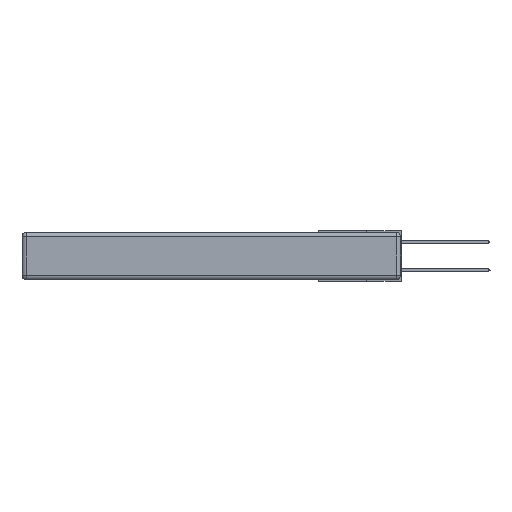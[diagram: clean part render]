
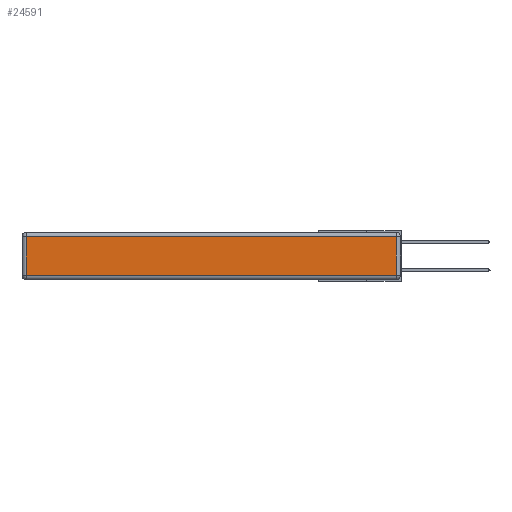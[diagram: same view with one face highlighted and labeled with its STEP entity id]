
A CAD part, left-side view. The second image highlights one B-rep face of the part: STEP entity #24591.
In plain terms, the highlighted planar face has unit normal (-1, 0, 0).
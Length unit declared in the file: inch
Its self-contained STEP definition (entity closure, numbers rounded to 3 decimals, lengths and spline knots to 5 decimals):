
#1178 = LINE ( 'NONE', #32410, #7089 ) ;
#2088 = CARTESIAN_POINT ( 'NONE',  ( 0., 0.03, -0.343 ) ) ;
#2269 = DIRECTION ( 'NONE',  ( 0., 0., -1. ) ) ;
#2375 = ORIENTED_EDGE ( 'NONE', *, *, #16801, .T. ) ;
#3249 = VERTEX_POINT ( 'NONE', #9468 ) ;
#5847 = DIRECTION ( 'NONE',  ( 0., 0., 1. ) ) ;
#6682 = DIRECTION ( 'NONE',  ( 0., -1., 0. ) ) ;
#7089 = VECTOR ( 'NONE', #22239, 39.37008 ) ;
#7823 = DIRECTION ( 'NONE',  ( -1., 0., 0. ) ) ;
#9468 = CARTESIAN_POINT ( 'NONE',  ( 0., 0.03, -0.313 ) ) ;
#9846 = EDGE_CURVE ( 'NONE', #3249, #24223, #26420, .T. ) ;
#10158 = VECTOR ( 'NONE', #27763, 39.37008 ) ;
#10250 = PLANE ( 'NONE',  #26780 ) ;
#10438 = EDGE_LOOP ( 'NONE', ( #25414, #20295, #2375, #22472 ) ) ;
#11338 = LINE ( 'NONE', #29591, #30744 ) ;
#11528 = LINE ( 'NONE', #15069, #28571 ) ;
#12261 = EDGE_CURVE ( 'NONE', #16256, #3249, #11338, .T. ) ;
#13826 = CARTESIAN_POINT ( 'NONE',  ( 0., 2.72, -0.03 ) ) ;
#15061 = CARTESIAN_POINT ( 'NONE',  ( 0., 2.72, -0.313 ) ) ;
#15069 = CARTESIAN_POINT ( 'NONE',  ( 0., 2.72, -0.343 ) ) ;
#16256 = VERTEX_POINT ( 'NONE', #15061 ) ;
#16801 = EDGE_CURVE ( 'NONE', #24223, #30823, #1178, .T. ) ;
#20295 = ORIENTED_EDGE ( 'NONE', *, *, #9846, .T. ) ;
#22239 = DIRECTION ( 'NONE',  ( 0., 1., 0. ) ) ;
#22472 = ORIENTED_EDGE ( 'NONE', *, *, #23863, .T. ) ;
#23811 = CARTESIAN_POINT ( 'NONE',  ( 0., 0.03, -0.03 ) ) ;
#23863 = EDGE_CURVE ( 'NONE', #30823, #16256, #11528, .T. ) ;
#24223 = VERTEX_POINT ( 'NONE', #23811 ) ;
#24591 = ADVANCED_FACE ( 'NONE', ( #32440 ), #10250, .T. ) ;
#25414 = ORIENTED_EDGE ( 'NONE', *, *, #12261, .T. ) ;
#26420 = LINE ( 'NONE', #2088, #10158 ) ;
#26780 = AXIS2_PLACEMENT_3D ( 'NONE', #27995, #7823, #5847 ) ;
#27763 = DIRECTION ( 'NONE',  ( 0., 0., 1. ) ) ;
#27995 = CARTESIAN_POINT ( 'NONE',  ( 0., 0., -0.343 ) ) ;
#28571 = VECTOR ( 'NONE', #2269, 39.37008 ) ;
#29591 = CARTESIAN_POINT ( 'NONE',  ( 0., 0., -0.313 ) ) ;
#30744 = VECTOR ( 'NONE', #6682, 39.37008 ) ;
#30823 = VERTEX_POINT ( 'NONE', #13826 ) ;
#32410 = CARTESIAN_POINT ( 'NONE',  ( 0., 2.75, -0.03 ) ) ;
#32440 = FACE_OUTER_BOUND ( 'NONE', #10438, .T. ) ;
